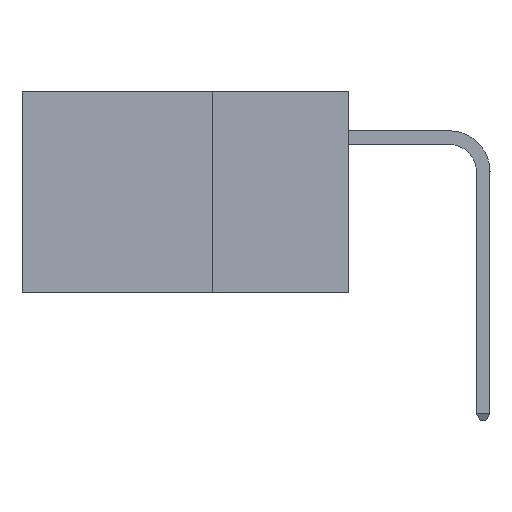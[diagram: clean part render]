
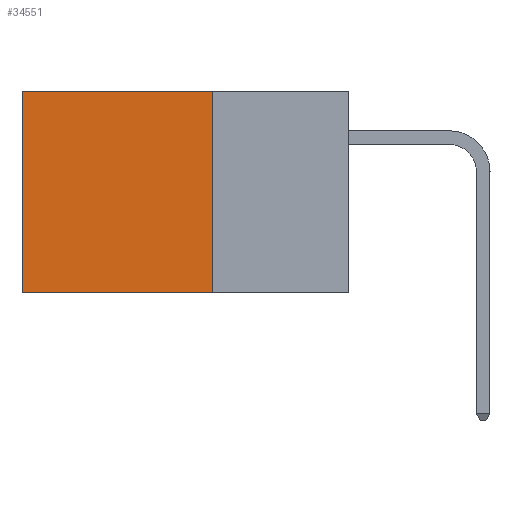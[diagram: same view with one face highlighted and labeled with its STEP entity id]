
A CAD part, left-side view. The second image highlights one B-rep face of the part: STEP entity #34551.
In plain terms, the highlighted planar face has unit normal (-1, 0, 0).
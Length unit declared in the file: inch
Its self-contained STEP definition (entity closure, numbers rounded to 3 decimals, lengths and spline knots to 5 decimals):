
#637 = CARTESIAN_POINT ( 'NONE',  ( 0.2875, 0.25, 0. ) ) ;
#3627 = DIRECTION ( 'NONE',  ( 0., 0., -1. ) ) ;
#4092 = EDGE_CURVE ( 'NONE', #34608, #27094, #35418, .T. ) ;
#5117 = DIRECTION ( 'NONE',  ( 0., 1., 0. ) ) ;
#8355 = EDGE_CURVE ( 'NONE', #34608, #12367, #10164, .T. ) ;
#8650 = EDGE_LOOP ( 'NONE', ( #20000, #33733, #38418, #36779 ) ) ;
#9849 = CARTESIAN_POINT ( 'NONE',  ( 0.2875, 0.25, 0. ) ) ;
#10164 = LINE ( 'NONE', #637, #24205 ) ;
#12367 = VERTEX_POINT ( 'NONE', #32369 ) ;
#13574 = CARTESIAN_POINT ( 'NONE',  ( 0.2875, 0.25, -0.37 ) ) ;
#14713 = CARTESIAN_POINT ( 'NONE',  ( 0.2875, 0.25, 0. ) ) ;
#18324 = CARTESIAN_POINT ( 'NONE',  ( 0.2875, 0.25, 0. ) ) ;
#18460 = DIRECTION ( 'NONE',  ( 1., 0., 0. ) ) ;
#20000 = ORIENTED_EDGE ( 'NONE', *, *, #33580, .T. ) ;
#20354 = CARTESIAN_POINT ( 'NONE',  ( 0.2875, 0.6, 0. ) ) ;
#21118 = DIRECTION ( 'NONE',  ( 0., 0., -1. ) ) ;
#23561 = EDGE_CURVE ( 'NONE', #27094, #23971, #30575, .T. ) ;
#23971 = VERTEX_POINT ( 'NONE', #32797 ) ;
#24205 = VECTOR ( 'NONE', #37181, 39.37008 ) ;
#24260 = VECTOR ( 'NONE', #28725, 39.37008 ) ;
#25437 = VECTOR ( 'NONE', #3627, 39.37008 ) ;
#27094 = VERTEX_POINT ( 'NONE', #13574 ) ;
#28725 = DIRECTION ( 'NONE',  ( 0., 0., -1. ) ) ;
#30575 = LINE ( 'NONE', #36918, #33566 ) ;
#32369 = CARTESIAN_POINT ( 'NONE',  ( 0.2875, 0.6, 0. ) ) ;
#32797 = CARTESIAN_POINT ( 'NONE',  ( 0.2875, 0.6, -0.37 ) ) ;
#33566 = VECTOR ( 'NONE', #5117, 39.37008 ) ;
#33580 = EDGE_CURVE ( 'NONE', #12367, #23971, #33743, .T. ) ;
#33733 = ORIENTED_EDGE ( 'NONE', *, *, #23561, .F. ) ;
#33743 = LINE ( 'NONE', #20354, #24260 ) ;
#34551 = ADVANCED_FACE ( 'NONE', ( #35131 ), #37656, .F. ) ;
#34608 = VERTEX_POINT ( 'NONE', #14713 ) ;
#35131 = FACE_OUTER_BOUND ( 'NONE', #8650, .T. ) ;
#35418 = LINE ( 'NONE', #9849, #25437 ) ;
#36779 = ORIENTED_EDGE ( 'NONE', *, *, #8355, .T. ) ;
#36918 = CARTESIAN_POINT ( 'NONE',  ( 0.2875, 0.25, -0.37 ) ) ;
#37181 = DIRECTION ( 'NONE',  ( 0., 1., 0. ) ) ;
#37350 = AXIS2_PLACEMENT_3D ( 'NONE', #18324, #18460, #21118 ) ;
#37656 = PLANE ( 'NONE',  #37350 ) ;
#38418 = ORIENTED_EDGE ( 'NONE', *, *, #4092, .F. ) ;
